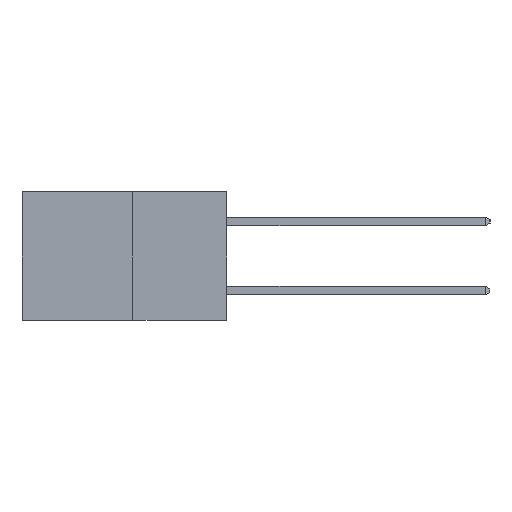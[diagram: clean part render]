
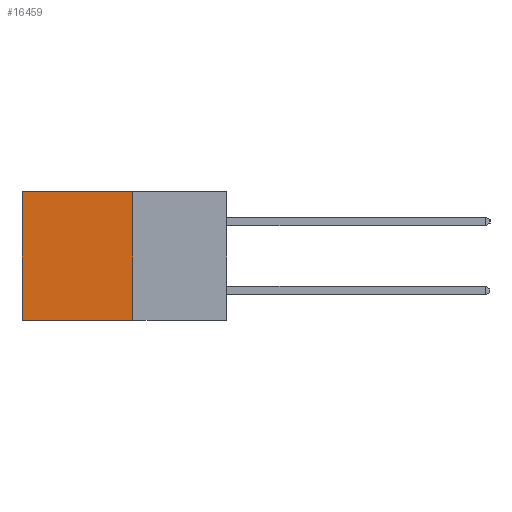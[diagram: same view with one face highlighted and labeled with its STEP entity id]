
A CAD part, left-side view. The second image highlights one B-rep face of the part: STEP entity #16459.
In plain terms, the highlighted planar face has unit normal (-1, 0, 0).
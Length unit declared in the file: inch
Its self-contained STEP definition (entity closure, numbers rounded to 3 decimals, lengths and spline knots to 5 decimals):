
#941 = EDGE_CURVE ( 'NONE', #8349, #4787, #5142, .T. ) ;
#1093 = DIRECTION ( 'NONE',  ( 1., 0., 0. ) ) ;
#1328 = VECTOR ( 'NONE', #1570, 39.37008 ) ;
#1521 = ORIENTED_EDGE ( 'NONE', *, *, #12634, .T. ) ;
#1570 = DIRECTION ( 'NONE',  ( 0., 1., 0. ) ) ;
#2542 = EDGE_CURVE ( 'NONE', #21017, #19350, #12975, .T. ) ;
#3165 = LINE ( 'NONE', #13924, #11336 ) ;
#3884 = CARTESIAN_POINT ( 'NONE',  ( 0.277, 0.27, -0.37 ) ) ;
#4051 = EDGE_LOOP ( 'NONE', ( #6937, #6955, #12715, #1521 ) ) ;
#4787 = VERTEX_POINT ( 'NONE', #10873 ) ;
#5142 = LINE ( 'NONE', #20777, #13306 ) ;
#6174 = AXIS2_PLACEMENT_3D ( 'NONE', #10915, #1093, #12537 ) ;
#6937 = ORIENTED_EDGE ( 'NONE', *, *, #941, .T. ) ;
#6955 = ORIENTED_EDGE ( 'NONE', *, *, #12359, .F. ) ;
#8349 = VERTEX_POINT ( 'NONE', #10786 ) ;
#10777 = FACE_OUTER_BOUND ( 'NONE', #4051, .T. ) ;
#10786 = CARTESIAN_POINT ( 'NONE',  ( 0.277, 0.59, 0. ) ) ;
#10845 = PLANE ( 'NONE',  #6174 ) ;
#10873 = CARTESIAN_POINT ( 'NONE',  ( 0.277, 0.59, -0.37 ) ) ;
#10915 = CARTESIAN_POINT ( 'NONE',  ( 0.277, 0.27, -0.37 ) ) ;
#11252 = DIRECTION ( 'NONE',  ( 0., 0., -1. ) ) ;
#11336 = VECTOR ( 'NONE', #13853, 39.37008 ) ;
#11742 = DIRECTION ( 'NONE',  ( 0., 0., -1. ) ) ;
#12114 = CARTESIAN_POINT ( 'NONE',  ( 0.277, 0.27, 0. ) ) ;
#12359 = EDGE_CURVE ( 'NONE', #19350, #4787, #3165, .T. ) ;
#12537 = DIRECTION ( 'NONE',  ( 0., 0., -1. ) ) ;
#12634 = EDGE_CURVE ( 'NONE', #21017, #8349, #14357, .T. ) ;
#12715 = ORIENTED_EDGE ( 'NONE', *, *, #2542, .F. ) ;
#12975 = LINE ( 'NONE', #3884, #20710 ) ;
#13306 = VECTOR ( 'NONE', #11742, 39.37008 ) ;
#13853 = DIRECTION ( 'NONE',  ( 0., 1., 0. ) ) ;
#13898 = CARTESIAN_POINT ( 'NONE',  ( 0.277, 0.27, -0.37 ) ) ;
#13924 = CARTESIAN_POINT ( 'NONE',  ( 0.277, 0.27, -0.37 ) ) ;
#14357 = LINE ( 'NONE', #21066, #1328 ) ;
#16459 = ADVANCED_FACE ( 'NONE', ( #10777 ), #10845, .F. ) ;
#19350 = VERTEX_POINT ( 'NONE', #13898 ) ;
#20710 = VECTOR ( 'NONE', #11252, 39.37008 ) ;
#20777 = CARTESIAN_POINT ( 'NONE',  ( 0.277, 0.59, -0.37 ) ) ;
#21017 = VERTEX_POINT ( 'NONE', #12114 ) ;
#21066 = CARTESIAN_POINT ( 'NONE',  ( 0.277, 0.27, 0. ) ) ;
